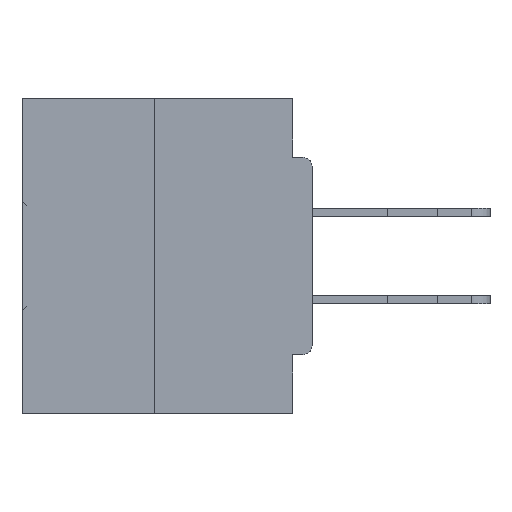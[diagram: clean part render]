
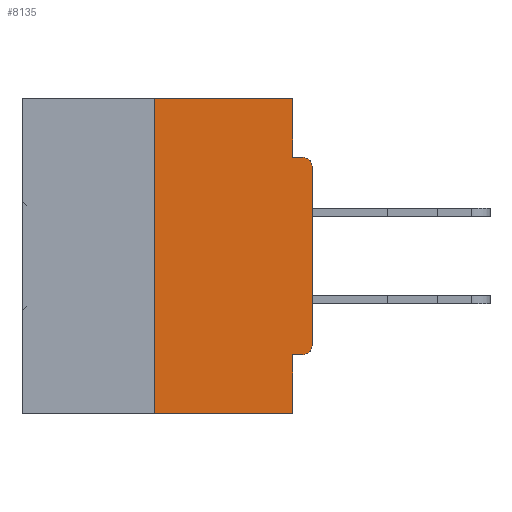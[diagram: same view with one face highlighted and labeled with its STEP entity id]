
A CAD part, left-side view. The second image highlights one B-rep face of the part: STEP entity #8135.
In plain terms, the highlighted planar face has unit normal (-1, 0, 0).
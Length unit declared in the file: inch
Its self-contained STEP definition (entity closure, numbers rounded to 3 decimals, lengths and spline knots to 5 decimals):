
#341 = CARTESIAN_POINT ( 'NONE',  ( 0., 0., -0.0935 ) ) ;
#2363 = AXIS2_PLACEMENT_3D ( 'NONE', #25826, #29381, #40551 ) ;
#2763 = VECTOR ( 'NONE', #26385, 39.37008 ) ;
#3307 = EDGE_CURVE ( 'NONE', #37883, #18119, #7221, .T. ) ;
#3329 = CARTESIAN_POINT ( 'NONE',  ( 0., 0.015, -0.1085 ) ) ;
#4035 = EDGE_CURVE ( 'NONE', #15967, #6120, #45400, .T. ) ;
#4448 = ORIENTED_EDGE ( 'NONE', *, *, #22339, .T. ) ;
#4686 = CARTESIAN_POINT ( 'NONE',  ( 0., 0., -0.4065 ) ) ;
#5292 = CARTESIAN_POINT ( 'NONE',  ( 0., 0.25, -0.5 ) ) ;
#5413 = CARTESIAN_POINT ( 'NONE',  ( 0., 0., -0.1085 ) ) ;
#5529 = CARTESIAN_POINT ( 'NONE',  ( 0., 0.031, -0.0935 ) ) ;
#5777 = CARTESIAN_POINT ( 'NONE',  ( 0., 0.031, -0.5 ) ) ;
#5782 = LINE ( 'NONE', #31624, #10802 ) ;
#5816 = CARTESIAN_POINT ( 'NONE',  ( 0., 0.46, 0. ) ) ;
#6120 = VERTEX_POINT ( 'NONE', #38204 ) ;
#6515 = CARTESIAN_POINT ( 'NONE',  ( 0., 0.46, -0.5 ) ) ;
#6907 = DIRECTION ( 'NONE',  ( 0., 0., -1. ) ) ;
#6951 = ORIENTED_EDGE ( 'NONE', *, *, #16031, .F. ) ;
#7030 = DIRECTION ( 'NONE',  ( 0., 0., -1. ) ) ;
#7221 = LINE ( 'NONE', #18840, #2763 ) ;
#7496 = DIRECTION ( 'NONE',  ( 0., -1., 0. ) ) ;
#7771 = LINE ( 'NONE', #28408, #9488 ) ;
#8135 = ADVANCED_FACE ( 'NONE', ( #36221 ), #45294, .F. ) ;
#8326 = EDGE_CURVE ( 'NONE', #10478, #23484, #5782, .T. ) ;
#8524 = ORIENTED_EDGE ( 'NONE', *, *, #36353, .T. ) ;
#9488 = VECTOR ( 'NONE', #31554, 39.37008 ) ;
#10445 = AXIS2_PLACEMENT_3D ( 'NONE', #5816, #27595, #31018 ) ;
#10478 = VERTEX_POINT ( 'NONE', #35791 ) ;
#10802 = VECTOR ( 'NONE', #7030, 39.37008 ) ;
#10922 = AXIS2_PLACEMENT_3D ( 'NONE', #3329, #28067, #6907 ) ;
#11193 = CARTESIAN_POINT ( 'NONE',  ( 0., 0., -0.3915 ) ) ;
#12683 = ORIENTED_EDGE ( 'NONE', *, *, #34760, .F. ) ;
#12882 = ORIENTED_EDGE ( 'NONE', *, *, #4035, .T. ) ;
#13210 = ORIENTED_EDGE ( 'NONE', *, *, #30724, .F. ) ;
#13450 = VECTOR ( 'NONE', #15077, 39.37008 ) ;
#13942 = VECTOR ( 'NONE', #7496, 39.37008 ) ;
#15077 = DIRECTION ( 'NONE',  ( 0., 0., -1. ) ) ;
#15202 = VERTEX_POINT ( 'NONE', #5777 ) ;
#15594 = VERTEX_POINT ( 'NONE', #11193 ) ;
#15967 = VERTEX_POINT ( 'NONE', #5413 ) ;
#16031 = EDGE_CURVE ( 'NONE', #18119, #10478, #7771, .T. ) ;
#16614 = LINE ( 'NONE', #27571, #40397 ) ;
#18119 = VERTEX_POINT ( 'NONE', #42678 ) ;
#18840 = CARTESIAN_POINT ( 'NONE',  ( 0., 0.25, 0. ) ) ;
#19155 = VECTOR ( 'NONE', #22617, 39.37008 ) ;
#20652 = LINE ( 'NONE', #36090, #13450 ) ;
#21913 = LINE ( 'NONE', #4686, #19155 ) ;
#22339 = EDGE_CURVE ( 'NONE', #15594, #15967, #16614, .T. ) ;
#22617 = DIRECTION ( 'NONE',  ( 0., 1., 0. ) ) ;
#23484 = VERTEX_POINT ( 'NONE', #5529 ) ;
#25826 = CARTESIAN_POINT ( 'NONE',  ( 0., 0.015, -0.3915 ) ) ;
#26385 = DIRECTION ( 'NONE',  ( 0., 0., 1. ) ) ;
#27571 = CARTESIAN_POINT ( 'NONE',  ( 0., 0., 0. ) ) ;
#27595 = DIRECTION ( 'NONE',  ( 1., 0., 0. ) ) ;
#28067 = DIRECTION ( 'NONE',  ( -1., 0., 0. ) ) ;
#28245 = ORIENTED_EDGE ( 'NONE', *, *, #35985, .T. ) ;
#28408 = CARTESIAN_POINT ( 'NONE',  ( 0., 0.46, 0. ) ) ;
#29381 = DIRECTION ( 'NONE',  ( -1., 0., 0. ) ) ;
#30724 = EDGE_CURVE ( 'NONE', #32034, #15202, #20652, .T. ) ;
#31018 = DIRECTION ( 'NONE',  ( 0., 0., -1. ) ) ;
#31554 = DIRECTION ( 'NONE',  ( 0., -1., 0. ) ) ;
#31560 = LINE ( 'NONE', #6515, #42624 ) ;
#31624 = CARTESIAN_POINT ( 'NONE',  ( 0., 0.031, 0. ) ) ;
#32034 = VERTEX_POINT ( 'NONE', #38824 ) ;
#32734 = LINE ( 'NONE', #341, #13942 ) ;
#34677 = DIRECTION ( 'NONE',  ( 0., 0., 1. ) ) ;
#34760 = EDGE_CURVE ( 'NONE', #23484, #6120, #32734, .T. ) ;
#35511 = EDGE_LOOP ( 'NONE', ( #6951, #45533, #28245, #13210, #38715, #8524, #4448, #12882, #12683, #36825 ) ) ;
#35791 = CARTESIAN_POINT ( 'NONE',  ( 0., 0.031, 0. ) ) ;
#35985 = EDGE_CURVE ( 'NONE', #37883, #15202, #31560, .T. ) ;
#36090 = CARTESIAN_POINT ( 'NONE',  ( 0., 0.031, -0.5 ) ) ;
#36221 = FACE_OUTER_BOUND ( 'NONE', #35511, .T. ) ;
#36353 = EDGE_CURVE ( 'NONE', #41758, #15594, #36487, .T. ) ;
#36487 = CIRCLE ( 'NONE', #2363, 0.015 ) ;
#36825 = ORIENTED_EDGE ( 'NONE', *, *, #8326, .F. ) ;
#37834 = CARTESIAN_POINT ( 'NONE',  ( 0., 0.015, -0.4065 ) ) ;
#37883 = VERTEX_POINT ( 'NONE', #5292 ) ;
#38204 = CARTESIAN_POINT ( 'NONE',  ( 0., 0.015, -0.0935 ) ) ;
#38715 = ORIENTED_EDGE ( 'NONE', *, *, #45867, .F. ) ;
#38824 = CARTESIAN_POINT ( 'NONE',  ( 0., 0.031, -0.4065 ) ) ;
#40397 = VECTOR ( 'NONE', #34677, 39.37008 ) ;
#40551 = DIRECTION ( 'NONE',  ( 0., 0., -1. ) ) ;
#41758 = VERTEX_POINT ( 'NONE', #37834 ) ;
#42624 = VECTOR ( 'NONE', #45238, 39.37008 ) ;
#42678 = CARTESIAN_POINT ( 'NONE',  ( 0., 0.25, 0. ) ) ;
#45238 = DIRECTION ( 'NONE',  ( 0., -1., 0. ) ) ;
#45294 = PLANE ( 'NONE',  #10445 ) ;
#45400 = CIRCLE ( 'NONE', #10922, 0.015 ) ;
#45533 = ORIENTED_EDGE ( 'NONE', *, *, #3307, .F. ) ;
#45867 = EDGE_CURVE ( 'NONE', #41758, #32034, #21913, .T. ) ;
